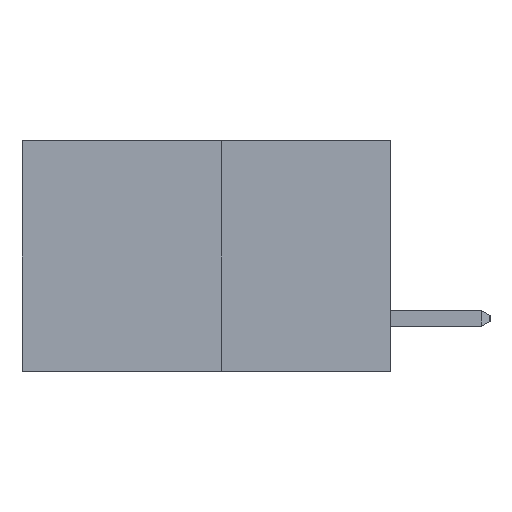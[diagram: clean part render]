
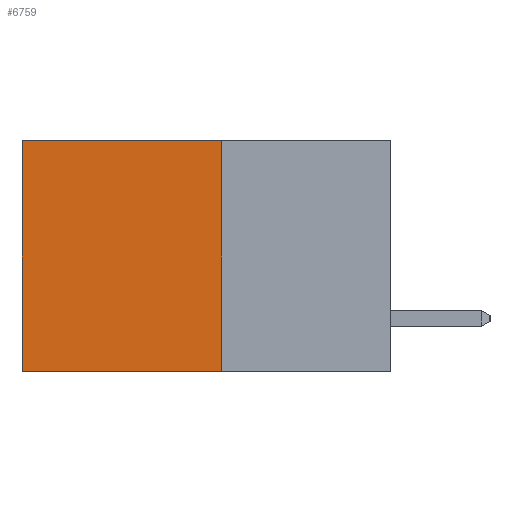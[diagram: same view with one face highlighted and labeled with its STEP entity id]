
A CAD part, left-side view. The second image highlights one B-rep face of the part: STEP entity #6759.
In plain terms, the highlighted planar face has unit normal (-1, 0, 0).
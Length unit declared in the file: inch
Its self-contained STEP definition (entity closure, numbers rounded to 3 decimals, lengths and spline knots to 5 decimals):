
#85 = ORIENTED_EDGE ( 'NONE', *, *, #4904, .T. ) ;
#451 = VECTOR ( 'NONE', #12481, 39.37008 ) ;
#926 = PLANE ( 'NONE',  #9735 ) ;
#1653 = FACE_OUTER_BOUND ( 'NONE', #7378, .T. ) ;
#1942 = DIRECTION ( 'NONE',  ( 0., 0., -1. ) ) ;
#2274 = LINE ( 'NONE', #2513, #11935 ) ;
#2513 = CARTESIAN_POINT ( 'NONE',  ( 0.277, 0.27, -0.37 ) ) ;
#3088 = VERTEX_POINT ( 'NONE', #8218 ) ;
#3239 = ORIENTED_EDGE ( 'NONE', *, *, #12170, .F. ) ;
#3451 = DIRECTION ( 'NONE',  ( 0., 0., -1. ) ) ;
#4904 = EDGE_CURVE ( 'NONE', #9842, #9100, #10091, .T. ) ;
#4905 = CARTESIAN_POINT ( 'NONE',  ( 0.277, 0.27, -0.37 ) ) ;
#4937 = ORIENTED_EDGE ( 'NONE', *, *, #7115, .F. ) ;
#5754 = LINE ( 'NONE', #7800, #451 ) ;
#6759 = ADVANCED_FACE ( 'NONE', ( #1653 ), #926, .F. ) ;
#6983 = DIRECTION ( 'NONE',  ( 0., 1., 0. ) ) ;
#7115 = EDGE_CURVE ( 'NONE', #11363, #3088, #2274, .T. ) ;
#7378 = EDGE_LOOP ( 'NONE', ( #11377, #4937, #3239, #85 ) ) ;
#7381 = CARTESIAN_POINT ( 'NONE',  ( 0.277, 0.27, 0. ) ) ;
#7580 = VECTOR ( 'NONE', #6983, 39.37008 ) ;
#7800 = CARTESIAN_POINT ( 'NONE',  ( 0.277, 0.27, -0.37 ) ) ;
#7875 = DIRECTION ( 'NONE',  ( 1., 0., 0. ) ) ;
#8130 = LINE ( 'NONE', #9293, #10024 ) ;
#8218 = CARTESIAN_POINT ( 'NONE',  ( 0.277, 0.59, -0.37 ) ) ;
#9100 = VERTEX_POINT ( 'NONE', #11038 ) ;
#9192 = EDGE_CURVE ( 'NONE', #9100, #3088, #8130, .T. ) ;
#9293 = CARTESIAN_POINT ( 'NONE',  ( 0.277, 0.59, -0.37 ) ) ;
#9735 = AXIS2_PLACEMENT_3D ( 'NONE', #4905, #7875, #1942 ) ;
#9842 = VERTEX_POINT ( 'NONE', #11173 ) ;
#9844 = CARTESIAN_POINT ( 'NONE',  ( 0.277, 0.27, -0.37 ) ) ;
#10024 = VECTOR ( 'NONE', #3451, 39.37008 ) ;
#10091 = LINE ( 'NONE', #7381, #7580 ) ;
#10276 = DIRECTION ( 'NONE',  ( 0., 1., 0. ) ) ;
#11038 = CARTESIAN_POINT ( 'NONE',  ( 0.277, 0.59, 0. ) ) ;
#11173 = CARTESIAN_POINT ( 'NONE',  ( 0.277, 0.27, 0. ) ) ;
#11363 = VERTEX_POINT ( 'NONE', #9844 ) ;
#11377 = ORIENTED_EDGE ( 'NONE', *, *, #9192, .T. ) ;
#11935 = VECTOR ( 'NONE', #10276, 39.37008 ) ;
#12170 = EDGE_CURVE ( 'NONE', #9842, #11363, #5754, .T. ) ;
#12481 = DIRECTION ( 'NONE',  ( 0., 0., -1. ) ) ;
